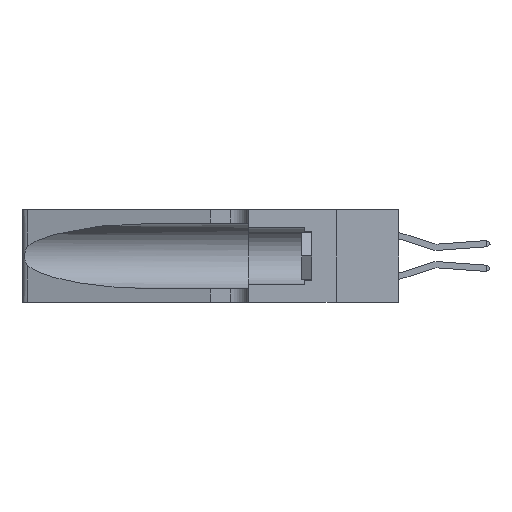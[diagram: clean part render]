
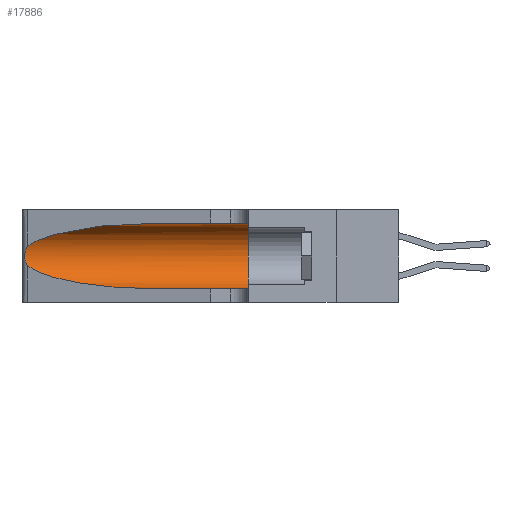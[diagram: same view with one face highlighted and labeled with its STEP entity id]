
A CAD part, left-side view. The second image highlights one B-rep face of the part: STEP entity #17886.
In plain terms, the highlighted cylindrical face has radius 3.308 mm (diameter 6.617 mm), a partial arc.
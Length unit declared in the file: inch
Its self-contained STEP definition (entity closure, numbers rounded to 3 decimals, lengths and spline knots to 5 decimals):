
#11 = CYLINDRICAL_SURFACE ( 'NONE', #10070, 0.13025 ) ;
#98 = EDGE_CURVE ( 'NONE', #3436, #40099, #4334, .T. ) ;
#523 = CARTESIAN_POINT ( 'NONE',  ( 0.18966, 0.96281, 0.05475 ) ) ;
#585 = CARTESIAN_POINT ( 'NONE',  ( 0.25854, 1.2359, 0.20912 ) ) ;
#2262 = CARTESIAN_POINT ( 'NONE',  ( 0.1305, 1.61858, 0.31525 ) ) ;
#3436 = VERTEX_POINT ( 'NONE', #30447 ) ;
#3603 = EDGE_CURVE ( 'NONE', #33025, #4668, #28071, .T. ) ;
#3661 =( BOUNDED_CURVE ( )  B_SPLINE_CURVE ( 3, ( #24041, #41014, #10435, #34346 ),
 .UNSPECIFIED., .F., .F. ) 
 B_SPLINE_CURVE_WITH_KNOTS ( ( 4, 4 ),
 ( 1.5708, 2.84003 ),
 .UNSPECIFIED. ) 
 CURVE ( )  GEOMETRIC_REPRESENTATION_ITEM ( )  RATIONAL_B_SPLINE_CURVE ( ( 1., 0.87, 0.87, 1. ) ) 
 REPRESENTATION_ITEM ( '' )  );
#3792 = ORIENTED_EDGE ( 'NONE', *, *, #36119, .T. ) ;
#3986 = CARTESIAN_POINT ( 'NONE',  ( 0.2373, 1.15595, 0.08982 ) ) ;
#4042 = CARTESIAN_POINT ( 'NONE',  ( 0.26075, 1.23896, 0.19203 ) ) ;
#4071 = B_SPLINE_CURVE_WITH_KNOTS ( 'NONE', 3,
 ( #31370, #10919, #41621, #21192, #585, #24654, #4042, #28112, #7551, #31519, #11068, #34947, #14499, #38352 ),
 .UNSPECIFIED., .F., .F.,
 ( 4, 2, 2, 2, 2, 2, 4 ),
 ( 0., 0.00027, 0.00053, 0.00107, 0.0016, 0.00187, 0.00214 ),
 .UNSPECIFIED. ) ;
#4216 = CARTESIAN_POINT ( 'NONE',  ( 0.1305, 1.61858, 0.185 ) ) ;
#4334 = LINE ( 'NONE', #2262, #13557 ) ;
#4619 = VERTEX_POINT ( 'NONE', #19711 ) ;
#4668 = VERTEX_POINT ( 'NONE', #16600 ) ;
#6177 = CARTESIAN_POINT ( 'NONE',  ( 0.1305, 0.35, 0.05475 ) ) ;
#7078 = ORIENTED_EDGE ( 'NONE', *, *, #98, .F. ) ;
#7495 = CARTESIAN_POINT ( 'NONE',  ( 0.1305, 0.72297, 0.05475 ) ) ;
#7551 = CARTESIAN_POINT ( 'NONE',  ( 0.26017, 1.23833, 0.17102 ) ) ;
#7725 = DIRECTION ( 'NONE',  ( 0., 0., -1. ) ) ;
#10070 = AXIS2_PLACEMENT_3D ( 'NONE', #4216, #28272, #7725 ) ;
#10435 = CARTESIAN_POINT ( 'NONE',  ( 0.2373, 1.15595, 0.28018 ) ) ;
#10919 = CARTESIAN_POINT ( 'NONE',  ( 0.25555, 1.22994, 0.2215 ) ) ;
#11068 = CARTESIAN_POINT ( 'NONE',  ( 0.25789, 1.23486, 0.15765 ) ) ;
#11871 = EDGE_CURVE ( 'NONE', #40099, #36843, #25165, .T. ) ;
#13557 = VECTOR ( 'NONE', #39879, 39.37008 ) ;
#13800 = VECTOR ( 'NONE', #26519, 39.37008 ) ;
#14499 = CARTESIAN_POINT ( 'NONE',  ( 0.25555, 1.22993, 0.14849 ) ) ;
#16574 = EDGE_CURVE ( 'NONE', #4619, #33025, #4071, .T. ) ;
#16600 = CARTESIAN_POINT ( 'NONE',  ( 0.1305, 0.72297, 0.05475 ) ) ;
#17457 = CARTESIAN_POINT ( 'NONE',  ( 0.1305, 0.35, 0.185 ) ) ;
#17886 = ADVANCED_FACE ( 'NONE', ( #36544 ), #11, .F. ) ;
#18340 = ORIENTED_EDGE ( 'NONE', *, *, #28477, .T. ) ;
#19711 = CARTESIAN_POINT ( 'NONE',  ( 0.25487, 1.22718, 0.22369 ) ) ;
#20890 = DIRECTION ( 'NONE',  ( 0., 0., 1. ) ) ;
#21192 = CARTESIAN_POINT ( 'NONE',  ( 0.25787, 1.23484, 0.2124 ) ) ;
#22105 = ORIENTED_EDGE ( 'NONE', *, *, #11871, .F. ) ;
#23930 = AXIS2_PLACEMENT_3D ( 'NONE', #17457, #41318, #20890 ) ;
#23936 = CARTESIAN_POINT ( 'NONE',  ( 0.25487, 1.22718, 0.14631 ) ) ;
#24041 = CARTESIAN_POINT ( 'NONE',  ( 0.1305, 0.72297, 0.31525 ) ) ;
#24654 = CARTESIAN_POINT ( 'NONE',  ( 0.26018, 1.23835, 0.19895 ) ) ;
#25165 = CIRCLE ( 'NONE', #23930, 0.13025 ) ;
#26519 = DIRECTION ( 'NONE',  ( 0., -1., 0. ) ) ;
#28054 = CARTESIAN_POINT ( 'NONE',  ( 0.25487, 1.22718, 0.14631 ) ) ;
#28071 =( BOUNDED_CURVE ( )  B_SPLINE_CURVE ( 3, ( #28054, #3986, #523, #7495 ),
 .UNSPECIFIED., .F., .T. ) 
 B_SPLINE_CURVE_WITH_KNOTS ( ( 4, 4 ),
 ( 3.44316, 4.71239 ),
 .UNSPECIFIED. ) 
 CURVE ( )  GEOMETRIC_REPRESENTATION_ITEM ( )  RATIONAL_B_SPLINE_CURVE ( ( 1., 0.87, 0.87, 1. ) ) 
 REPRESENTATION_ITEM ( '' )  );
#28112 = CARTESIAN_POINT ( 'NONE',  ( 0.26075, 1.23896, 0.178 ) ) ;
#28272 = DIRECTION ( 'NONE',  ( 0., -1., 0. ) ) ;
#28477 = EDGE_CURVE ( 'NONE', #3436, #4619, #3661, .T. ) ;
#30447 = CARTESIAN_POINT ( 'NONE',  ( 0.1305, 0.72297, 0.31525 ) ) ;
#31370 = CARTESIAN_POINT ( 'NONE',  ( 0.25487, 1.22718, 0.22369 ) ) ;
#31519 = CARTESIAN_POINT ( 'NONE',  ( 0.25856, 1.23593, 0.16098 ) ) ;
#33025 = VERTEX_POINT ( 'NONE', #23936 ) ;
#34346 = CARTESIAN_POINT ( 'NONE',  ( 0.25487, 1.22718, 0.22369 ) ) ;
#34947 = CARTESIAN_POINT ( 'NONE',  ( 0.25639, 1.23186, 0.15144 ) ) ;
#36119 = EDGE_CURVE ( 'NONE', #4668, #36843, #43135, .T. ) ;
#36544 = FACE_OUTER_BOUND ( 'NONE', #38712, .T. ) ;
#36843 = VERTEX_POINT ( 'NONE', #6177 ) ;
#37057 = ORIENTED_EDGE ( 'NONE', *, *, #3603, .T. ) ;
#37955 = CARTESIAN_POINT ( 'NONE',  ( 0.1305, 0.35, 0.31525 ) ) ;
#38352 = CARTESIAN_POINT ( 'NONE',  ( 0.25487, 1.22718, 0.14631 ) ) ;
#38622 = ORIENTED_EDGE ( 'NONE', *, *, #16574, .T. ) ;
#38712 = EDGE_LOOP ( 'NONE', ( #18340, #38622, #37057, #3792, #22105, #7078 ) ) ;
#39879 = DIRECTION ( 'NONE',  ( 0., -1., 0. ) ) ;
#40099 = VERTEX_POINT ( 'NONE', #37955 ) ;
#41014 = CARTESIAN_POINT ( 'NONE',  ( 0.18966, 0.96281, 0.31525 ) ) ;
#41318 = DIRECTION ( 'NONE',  ( 0., 1., 0. ) ) ;
#41621 = CARTESIAN_POINT ( 'NONE',  ( 0.25639, 1.23184, 0.21858 ) ) ;
#43135 = LINE ( 'NONE', #43472, #13800 ) ;
#43472 = CARTESIAN_POINT ( 'NONE',  ( 0.1305, 1.61858, 0.05475 ) ) ;
